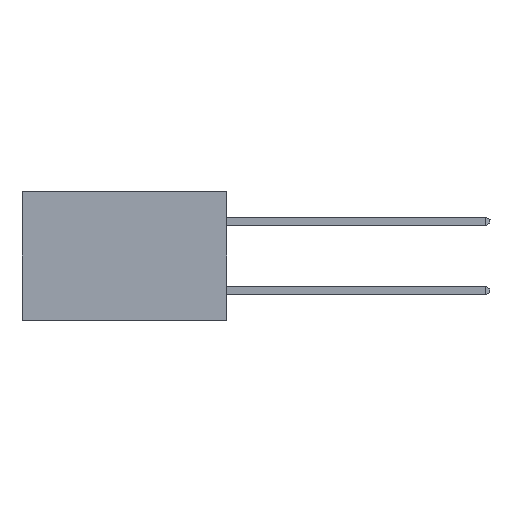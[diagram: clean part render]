
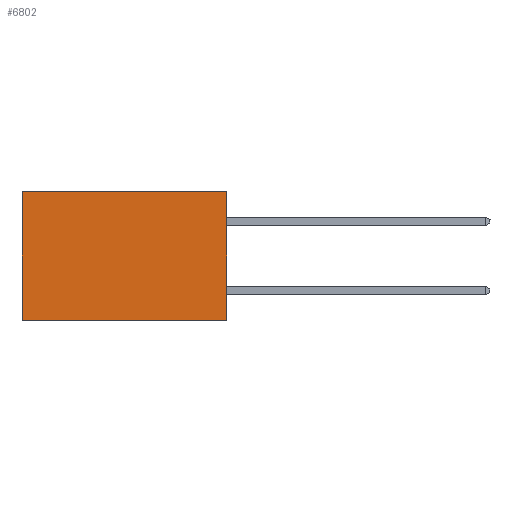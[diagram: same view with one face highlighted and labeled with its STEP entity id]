
A CAD part, left-side view. The second image highlights one B-rep face of the part: STEP entity #6802.
In plain terms, the highlighted planar face has unit normal (-1, 0, 0).
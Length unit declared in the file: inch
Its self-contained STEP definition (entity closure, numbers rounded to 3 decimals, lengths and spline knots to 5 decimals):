
#430 = ORIENTED_EDGE ( 'NONE', *, *, #5618, .T. ) ;
#748 = AXIS2_PLACEMENT_3D ( 'NONE', #8020, #6762, #2767 ) ;
#837 = DIRECTION ( 'NONE',  ( 0., 1., 0. ) ) ;
#896 = VERTEX_POINT ( 'NONE', #7977 ) ;
#1272 = EDGE_CURVE ( 'NONE', #896, #4427, #3775, .T. ) ;
#1406 = LINE ( 'NONE', #4321, #2550 ) ;
#1545 = DIRECTION ( 'NONE',  ( 0., 1., 0. ) ) ;
#1682 = CARTESIAN_POINT ( 'NONE',  ( 0.277, 0., 0. ) ) ;
#1796 = EDGE_CURVE ( 'NONE', #4222, #7865, #2414, .T. ) ;
#2005 = VECTOR ( 'NONE', #1545, 39.37008 ) ;
#2414 = LINE ( 'NONE', #8567, #6201 ) ;
#2550 = VECTOR ( 'NONE', #7011, 39.37008 ) ;
#2767 = DIRECTION ( 'NONE',  ( 0., 0., -1. ) ) ;
#2919 = CARTESIAN_POINT ( 'NONE',  ( 0.277, 0., -0.37 ) ) ;
#3775 = LINE ( 'NONE', #1682, #2005 ) ;
#4026 = ORIENTED_EDGE ( 'NONE', *, *, #1796, .F. ) ;
#4222 = VERTEX_POINT ( 'NONE', #2919 ) ;
#4321 = CARTESIAN_POINT ( 'NONE',  ( 0.277, 0., -0.37 ) ) ;
#4427 = VERTEX_POINT ( 'NONE', #7493 ) ;
#4864 = ORIENTED_EDGE ( 'NONE', *, *, #8586, .F. ) ;
#5066 = ORIENTED_EDGE ( 'NONE', *, *, #1272, .T. ) ;
#5238 = DIRECTION ( 'NONE',  ( 0., 0., -1. ) ) ;
#5416 = PLANE ( 'NONE',  #748 ) ;
#5618 = EDGE_CURVE ( 'NONE', #4427, #7865, #6169, .T. ) ;
#5958 = VECTOR ( 'NONE', #5238, 39.37008 ) ;
#6169 = LINE ( 'NONE', #7901, #5958 ) ;
#6201 = VECTOR ( 'NONE', #837, 39.37008 ) ;
#6762 = DIRECTION ( 'NONE',  ( 1., 0., 0. ) ) ;
#6802 = ADVANCED_FACE ( 'NONE', ( #7076 ), #5416, .F. ) ;
#6816 = EDGE_LOOP ( 'NONE', ( #430, #4026, #4864, #5066 ) ) ;
#7011 = DIRECTION ( 'NONE',  ( 0., 0., -1. ) ) ;
#7076 = FACE_OUTER_BOUND ( 'NONE', #6816, .T. ) ;
#7081 = CARTESIAN_POINT ( 'NONE',  ( 0.277, 0.59, -0.37 ) ) ;
#7493 = CARTESIAN_POINT ( 'NONE',  ( 0.277, 0.59, 0. ) ) ;
#7865 = VERTEX_POINT ( 'NONE', #7081 ) ;
#7901 = CARTESIAN_POINT ( 'NONE',  ( 0.277, 0.59, -0.37 ) ) ;
#7977 = CARTESIAN_POINT ( 'NONE',  ( 0.277, 0., 0. ) ) ;
#8020 = CARTESIAN_POINT ( 'NONE',  ( 0.277, 0., -0.37 ) ) ;
#8567 = CARTESIAN_POINT ( 'NONE',  ( 0.277, 0., -0.37 ) ) ;
#8586 = EDGE_CURVE ( 'NONE', #896, #4222, #1406, .T. ) ;
